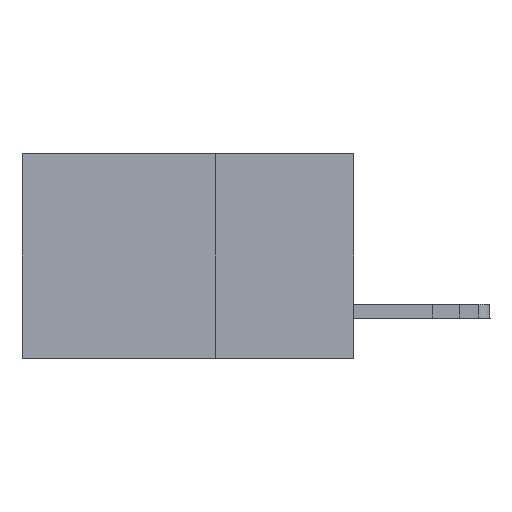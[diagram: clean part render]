
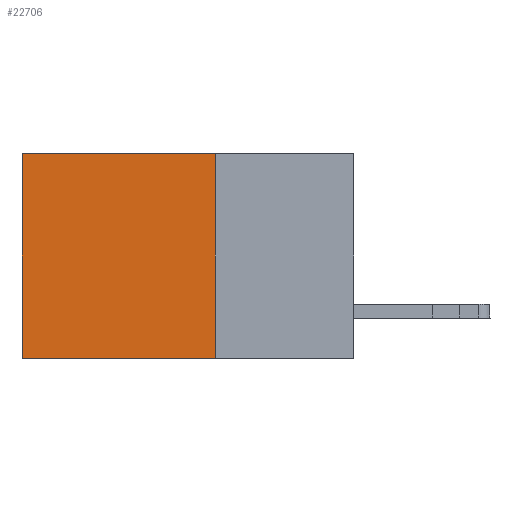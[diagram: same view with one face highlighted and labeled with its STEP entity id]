
A CAD part, left-side view. The second image highlights one B-rep face of the part: STEP entity #22706.
In plain terms, the highlighted planar face has unit normal (-1, 0, 0).
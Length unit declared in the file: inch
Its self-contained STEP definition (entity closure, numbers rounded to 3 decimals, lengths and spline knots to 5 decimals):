
#56 = EDGE_CURVE ( 'NONE', #14834, #23210, #27150, .T. ) ;
#1004 = VERTEX_POINT ( 'NONE', #26662 ) ;
#1561 = ORIENTED_EDGE ( 'NONE', *, *, #18052, .T. ) ;
#4136 = DIRECTION ( 'NONE',  ( 1., 0., 0. ) ) ;
#4923 = CARTESIAN_POINT ( 'NONE',  ( 0.2875, 0.25, 0. ) ) ;
#5818 = DIRECTION ( 'NONE',  ( 0., 0., -1. ) ) ;
#6672 = CARTESIAN_POINT ( 'NONE',  ( 0.2875, 0.6, 0. ) ) ;
#6694 = EDGE_CURVE ( 'NONE', #10758, #1004, #18866, .T. ) ;
#7838 = CARTESIAN_POINT ( 'NONE',  ( 0.2875, 0.6, -0.37 ) ) ;
#8811 = CARTESIAN_POINT ( 'NONE',  ( 0.2875, 0.25, -0.37 ) ) ;
#9251 = LINE ( 'NONE', #4923, #14074 ) ;
#9514 = AXIS2_PLACEMENT_3D ( 'NONE', #18626, #4136, #18715 ) ;
#10353 = VECTOR ( 'NONE', #10889, 39.37008 ) ;
#10599 = EDGE_CURVE ( 'NONE', #1004, #23210, #15845, .T. ) ;
#10758 = VERTEX_POINT ( 'NONE', #23888 ) ;
#10889 = DIRECTION ( 'NONE',  ( 0., 1., 0. ) ) ;
#11898 = FACE_OUTER_BOUND ( 'NONE', #22330, .T. ) ;
#12056 = CARTESIAN_POINT ( 'NONE',  ( 0.2875, 0.25, 0. ) ) ;
#12058 = ORIENTED_EDGE ( 'NONE', *, *, #6694, .F. ) ;
#12233 = DIRECTION ( 'NONE',  ( 0., 0., -1. ) ) ;
#12431 = CARTESIAN_POINT ( 'NONE',  ( 0.2875, 0.6, 0. ) ) ;
#13201 = ORIENTED_EDGE ( 'NONE', *, *, #56, .T. ) ;
#14074 = VECTOR ( 'NONE', #17543, 39.37008 ) ;
#14834 = VERTEX_POINT ( 'NONE', #6672 ) ;
#15845 = LINE ( 'NONE', #8811, #10353 ) ;
#16609 = PLANE ( 'NONE',  #9514 ) ;
#17543 = DIRECTION ( 'NONE',  ( 0., 1., 0. ) ) ;
#18052 = EDGE_CURVE ( 'NONE', #10758, #14834, #9251, .T. ) ;
#18626 = CARTESIAN_POINT ( 'NONE',  ( 0.2875, 0.25, 0. ) ) ;
#18715 = DIRECTION ( 'NONE',  ( 0., 0., -1. ) ) ;
#18866 = LINE ( 'NONE', #12056, #23777 ) ;
#22330 = EDGE_LOOP ( 'NONE', ( #13201, #26100, #12058, #1561 ) ) ;
#22706 = ADVANCED_FACE ( 'NONE', ( #11898 ), #16609, .F. ) ;
#23210 = VERTEX_POINT ( 'NONE', #7838 ) ;
#23550 = VECTOR ( 'NONE', #12233, 39.37008 ) ;
#23777 = VECTOR ( 'NONE', #5818, 39.37008 ) ;
#23888 = CARTESIAN_POINT ( 'NONE',  ( 0.2875, 0.25, 0. ) ) ;
#26100 = ORIENTED_EDGE ( 'NONE', *, *, #10599, .F. ) ;
#26662 = CARTESIAN_POINT ( 'NONE',  ( 0.2875, 0.25, -0.37 ) ) ;
#27150 = LINE ( 'NONE', #12431, #23550 ) ;
